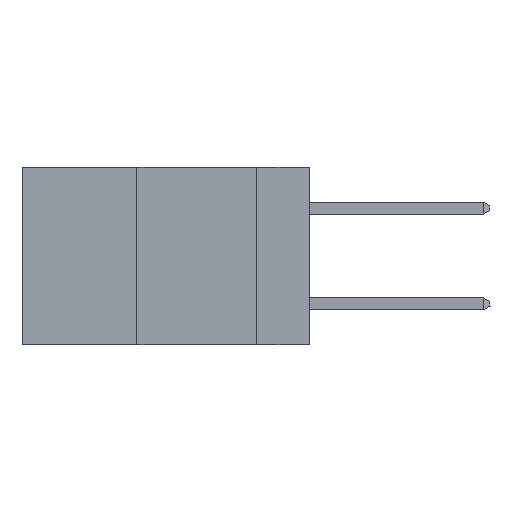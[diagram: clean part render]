
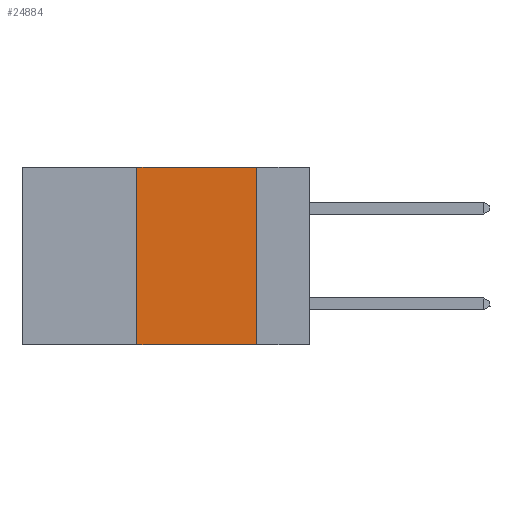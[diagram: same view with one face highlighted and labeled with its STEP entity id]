
A CAD part, left-side view. The second image highlights one B-rep face of the part: STEP entity #24884.
In plain terms, the highlighted planar face has unit normal (-1, 0, 0).
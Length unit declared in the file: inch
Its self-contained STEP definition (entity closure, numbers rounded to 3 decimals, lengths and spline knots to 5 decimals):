
#193 = VECTOR ( 'NONE', #9918, 39.37008 ) ;
#1920 = EDGE_CURVE ( 'NONE', #4548, #3788, #23365, .T. ) ;
#2205 = CARTESIAN_POINT ( 'NONE',  ( 0., 0.36, 0. ) ) ;
#3617 = ORIENTED_EDGE ( 'NONE', *, *, #13175, .F. ) ;
#3788 = VERTEX_POINT ( 'NONE', #13041 ) ;
#4462 = LINE ( 'NONE', #15894, #8071 ) ;
#4548 = VERTEX_POINT ( 'NONE', #2205 ) ;
#4639 = VERTEX_POINT ( 'NONE', #16655 ) ;
#5220 = DIRECTION ( 'NONE',  ( 0., 0., 1. ) ) ;
#7003 = LINE ( 'NONE', #20592, #13247 ) ;
#8071 = VECTOR ( 'NONE', #14007, 39.37008 ) ;
#8734 = ORIENTED_EDGE ( 'NONE', *, *, #23976, .T. ) ;
#9918 = DIRECTION ( 'NONE',  ( 0., -1., 0. ) ) ;
#10214 = PLANE ( 'NONE',  #14582 ) ;
#11031 = CARTESIAN_POINT ( 'NONE',  ( 0., 0.11, 0. ) ) ;
#11284 = DIRECTION ( 'NONE',  ( 0., 0., -1. ) ) ;
#11955 = CARTESIAN_POINT ( 'NONE',  ( 0., 0.11, -0.37 ) ) ;
#12377 = VECTOR ( 'NONE', #11284, 39.37008 ) ;
#13041 = CARTESIAN_POINT ( 'NONE',  ( 0., 0.11, 0. ) ) ;
#13175 = EDGE_CURVE ( 'NONE', #4639, #4548, #7003, .T. ) ;
#13247 = VECTOR ( 'NONE', #5220, 39.37008 ) ;
#13999 = VERTEX_POINT ( 'NONE', #11955 ) ;
#14007 = DIRECTION ( 'NONE',  ( 0., -1., 0. ) ) ;
#14582 = AXIS2_PLACEMENT_3D ( 'NONE', #19636, #19754, #17844 ) ;
#15464 = ORIENTED_EDGE ( 'NONE', *, *, #1920, .F. ) ;
#15790 = EDGE_CURVE ( 'NONE', #3788, #13999, #24737, .T. ) ;
#15811 = FACE_OUTER_BOUND ( 'NONE', #18075, .T. ) ;
#15894 = CARTESIAN_POINT ( 'NONE',  ( 0., 0.6, -0.37 ) ) ;
#16307 = ORIENTED_EDGE ( 'NONE', *, *, #15790, .F. ) ;
#16655 = CARTESIAN_POINT ( 'NONE',  ( 0., 0.36, -0.37 ) ) ;
#17844 = DIRECTION ( 'NONE',  ( 0., 0., -1. ) ) ;
#18075 = EDGE_LOOP ( 'NONE', ( #16307, #15464, #3617, #8734 ) ) ;
#19636 = CARTESIAN_POINT ( 'NONE',  ( 0., 0.6, 0. ) ) ;
#19754 = DIRECTION ( 'NONE',  ( 1., 0., 0. ) ) ;
#20592 = CARTESIAN_POINT ( 'NONE',  ( 0., 0.36, 0. ) ) ;
#23365 = LINE ( 'NONE', #25024, #193 ) ;
#23976 = EDGE_CURVE ( 'NONE', #4639, #13999, #4462, .T. ) ;
#24737 = LINE ( 'NONE', #11031, #12377 ) ;
#24884 = ADVANCED_FACE ( 'NONE', ( #15811 ), #10214, .F. ) ;
#25024 = CARTESIAN_POINT ( 'NONE',  ( 0., 0.6, 0. ) ) ;
